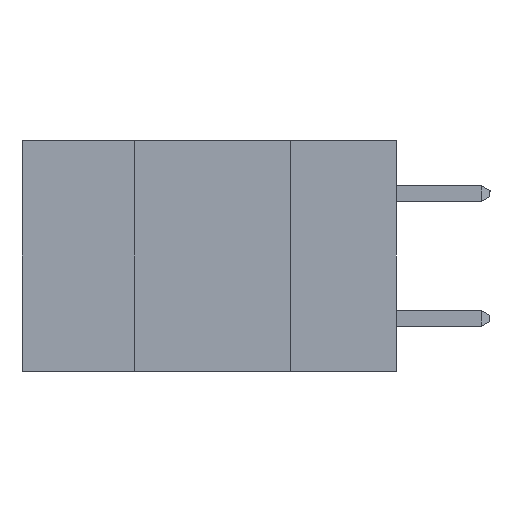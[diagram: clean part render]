
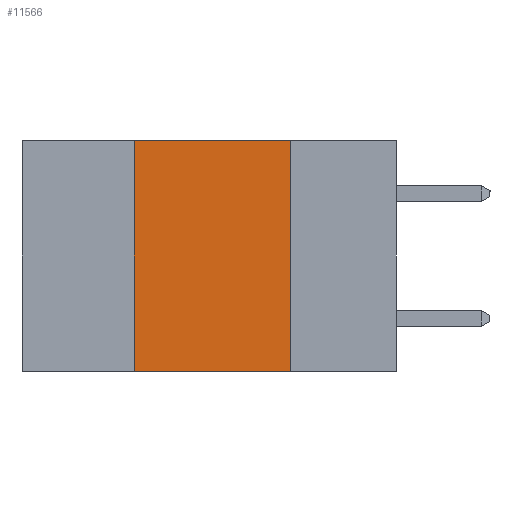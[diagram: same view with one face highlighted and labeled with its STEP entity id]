
A CAD part, left-side view. The second image highlights one B-rep face of the part: STEP entity #11566.
In plain terms, the highlighted planar face has unit normal (-1, 0, 0).
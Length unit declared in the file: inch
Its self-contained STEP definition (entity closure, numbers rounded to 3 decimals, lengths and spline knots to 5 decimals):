
#406 = CARTESIAN_POINT ( 'NONE',  ( 0., 0.17, -0.37 ) ) ;
#691 = DIRECTION ( 'NONE',  ( 0., -1., 0. ) ) ;
#1080 = VERTEX_POINT ( 'NONE', #406 ) ;
#1400 = DIRECTION ( 'NONE',  ( 0., 0., -1. ) ) ;
#2015 = CARTESIAN_POINT ( 'NONE',  ( 0., 0.17, -0.37 ) ) ;
#2292 = CARTESIAN_POINT ( 'NONE',  ( 0., 0.6, 0. ) ) ;
#3057 = VECTOR ( 'NONE', #4986, 39.37008 ) ;
#3070 = EDGE_CURVE ( 'NONE', #8975, #17995, #13351, .T. ) ;
#3132 = PLANE ( 'NONE',  #4646 ) ;
#3653 = LINE ( 'NONE', #2015, #11919 ) ;
#4485 = CARTESIAN_POINT ( 'NONE',  ( 0., 0.42, -0.37 ) ) ;
#4646 = AXIS2_PLACEMENT_3D ( 'NONE', #14591, #14682, #1400 ) ;
#4792 = VECTOR ( 'NONE', #10760, 39.37008 ) ;
#4986 = DIRECTION ( 'NONE',  ( 0., -1., 0. ) ) ;
#5494 = CARTESIAN_POINT ( 'NONE',  ( 0., 0.6, -0.37 ) ) ;
#5673 = CARTESIAN_POINT ( 'NONE',  ( 0., 0.42, 0. ) ) ;
#6269 = VERTEX_POINT ( 'NONE', #8391 ) ;
#6918 = LINE ( 'NONE', #5494, #8873 ) ;
#7153 = ORIENTED_EDGE ( 'NONE', *, *, #8108, .T. ) ;
#7174 = EDGE_CURVE ( 'NONE', #17995, #6269, #9609, .T. ) ;
#7247 = ORIENTED_EDGE ( 'NONE', *, *, #15087, .F. ) ;
#8070 = DIRECTION ( 'NONE',  ( 0., 0., -1. ) ) ;
#8108 = EDGE_CURVE ( 'NONE', #8975, #1080, #6918, .T. ) ;
#8391 = CARTESIAN_POINT ( 'NONE',  ( 0., 0.17, 0. ) ) ;
#8795 = FACE_OUTER_BOUND ( 'NONE', #11383, .T. ) ;
#8873 = VECTOR ( 'NONE', #691, 39.37008 ) ;
#8975 = VERTEX_POINT ( 'NONE', #15934 ) ;
#9609 = LINE ( 'NONE', #2292, #3057 ) ;
#10760 = DIRECTION ( 'NONE',  ( 0., 0., 1. ) ) ;
#11383 = EDGE_LOOP ( 'NONE', ( #7247, #14512, #15058, #7153 ) ) ;
#11566 = ADVANCED_FACE ( 'NONE', ( #8795 ), #3132, .F. ) ;
#11919 = VECTOR ( 'NONE', #8070, 39.37008 ) ;
#13351 = LINE ( 'NONE', #4485, #4792 ) ;
#14512 = ORIENTED_EDGE ( 'NONE', *, *, #7174, .F. ) ;
#14591 = CARTESIAN_POINT ( 'NONE',  ( 0., 0.6, 0. ) ) ;
#14682 = DIRECTION ( 'NONE',  ( 1., 0., 0. ) ) ;
#15058 = ORIENTED_EDGE ( 'NONE', *, *, #3070, .F. ) ;
#15087 = EDGE_CURVE ( 'NONE', #6269, #1080, #3653, .T. ) ;
#15934 = CARTESIAN_POINT ( 'NONE',  ( 0., 0.42, -0.37 ) ) ;
#17995 = VERTEX_POINT ( 'NONE', #5673 ) ;
